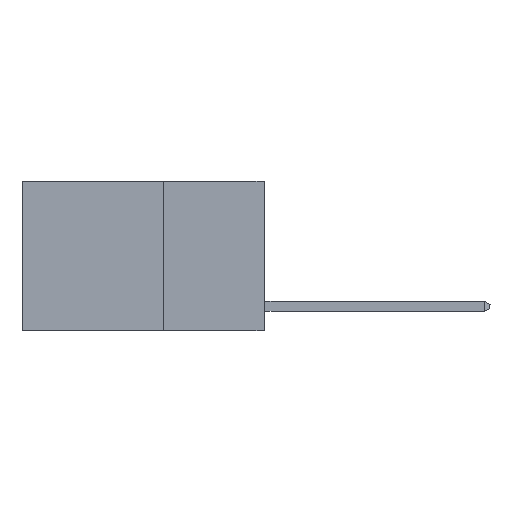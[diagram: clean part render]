
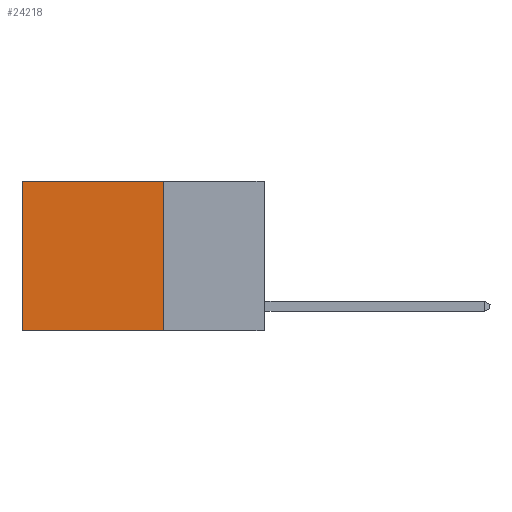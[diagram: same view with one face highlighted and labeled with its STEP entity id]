
A CAD part, left-side view. The second image highlights one B-rep face of the part: STEP entity #24218.
In plain terms, the highlighted planar face has unit normal (-1, 0, 0).
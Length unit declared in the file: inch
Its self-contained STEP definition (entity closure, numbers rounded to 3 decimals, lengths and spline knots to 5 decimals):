
#391 = EDGE_LOOP ( 'NONE', ( #20080, #2356, #20774, #4581 ) ) ;
#1759 = DIRECTION ( 'NONE',  ( 0., 0., -1. ) ) ;
#2356 = ORIENTED_EDGE ( 'NONE', *, *, #8477, .F. ) ;
#3419 = VERTEX_POINT ( 'NONE', #23211 ) ;
#4110 = FACE_OUTER_BOUND ( 'NONE', #391, .T. ) ;
#4581 = ORIENTED_EDGE ( 'NONE', *, *, #9969, .T. ) ;
#6598 = LINE ( 'NONE', #21946, #11969 ) ;
#8477 = EDGE_CURVE ( 'NONE', #9157, #23721, #9253, .T. ) ;
#9157 = VERTEX_POINT ( 'NONE', #20238 ) ;
#9253 = LINE ( 'NONE', #24705, #25158 ) ;
#9969 = EDGE_CURVE ( 'NONE', #3419, #21290, #25455, .T. ) ;
#10975 = PLANE ( 'NONE',  #25524 ) ;
#11182 = CARTESIAN_POINT ( 'NONE',  ( 0.2625, 0.6, -0.37 ) ) ;
#11969 = VECTOR ( 'NONE', #28705, 39.37008 ) ;
#12625 = VECTOR ( 'NONE', #18403, 39.37008 ) ;
#13239 = CARTESIAN_POINT ( 'NONE',  ( 0.2625, 0.25, 0. ) ) ;
#13334 = LINE ( 'NONE', #16153, #12625 ) ;
#13478 = VECTOR ( 'NONE', #20683, 39.37008 ) ;
#15537 = DIRECTION ( 'NONE',  ( 1., 0., 0. ) ) ;
#16153 = CARTESIAN_POINT ( 'NONE',  ( 0.2625, 0.25, 0. ) ) ;
#17614 = CARTESIAN_POINT ( 'NONE',  ( 0.2625, 0.6, 0. ) ) ;
#17635 = EDGE_CURVE ( 'NONE', #21290, #23721, #6598, .T. ) ;
#18400 = CARTESIAN_POINT ( 'NONE',  ( 0.2625, 0.25, 0. ) ) ;
#18403 = DIRECTION ( 'NONE',  ( 0., 0., -1. ) ) ;
#19118 = EDGE_CURVE ( 'NONE', #3419, #9157, #13334, .T. ) ;
#20080 = ORIENTED_EDGE ( 'NONE', *, *, #17635, .T. ) ;
#20238 = CARTESIAN_POINT ( 'NONE',  ( 0.2625, 0.25, -0.37 ) ) ;
#20683 = DIRECTION ( 'NONE',  ( 0., 1., 0. ) ) ;
#20774 = ORIENTED_EDGE ( 'NONE', *, *, #19118, .F. ) ;
#21290 = VERTEX_POINT ( 'NONE', #17614 ) ;
#21946 = CARTESIAN_POINT ( 'NONE',  ( 0.2625, 0.6, 0. ) ) ;
#22530 = DIRECTION ( 'NONE',  ( 0., 1., 0. ) ) ;
#23211 = CARTESIAN_POINT ( 'NONE',  ( 0.2625, 0.25, 0. ) ) ;
#23721 = VERTEX_POINT ( 'NONE', #11182 ) ;
#24218 = ADVANCED_FACE ( 'NONE', ( #4110 ), #10975, .F. ) ;
#24705 = CARTESIAN_POINT ( 'NONE',  ( 0.2625, 0.25, -0.37 ) ) ;
#25158 = VECTOR ( 'NONE', #22530, 39.37008 ) ;
#25455 = LINE ( 'NONE', #18400, #13478 ) ;
#25524 = AXIS2_PLACEMENT_3D ( 'NONE', #13239, #15537, #1759 ) ;
#28705 = DIRECTION ( 'NONE',  ( 0., 0., -1. ) ) ;
